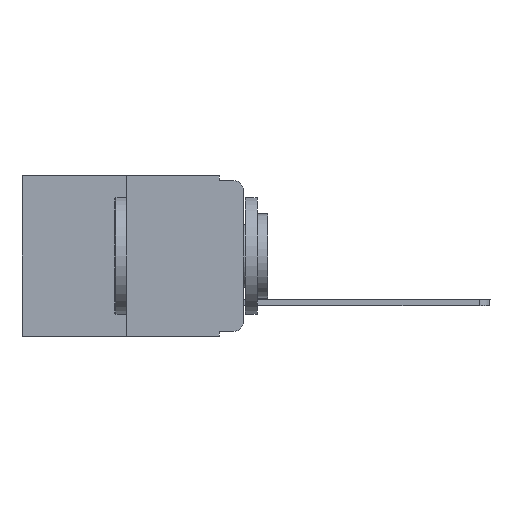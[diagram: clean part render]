
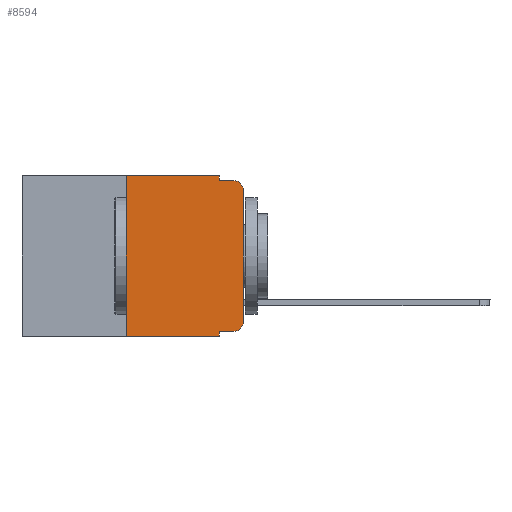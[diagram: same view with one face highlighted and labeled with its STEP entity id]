
A CAD part, left-side view. The second image highlights one B-rep face of the part: STEP entity #8594.
In plain terms, the highlighted planar face has unit normal (-1, 0, 0).
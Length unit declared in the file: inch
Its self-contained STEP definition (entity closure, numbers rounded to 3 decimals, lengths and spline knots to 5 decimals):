
#75 = EDGE_CURVE ( 'NONE', #5653, #9041, #9872, .T. ) ;
#121 = VECTOR ( 'NONE', #3713, 39.37008 ) ;
#231 = CARTESIAN_POINT ( 'NONE',  ( 0., 0.473, 0. ) ) ;
#342 = LINE ( 'NONE', #6228, #9351 ) ;
#469 = LINE ( 'NONE', #10474, #3541 ) ;
#540 = EDGE_LOOP ( 'NONE', ( #1932, #5531, #7216, #6764, #4128, #2574, #12078, #12370, #7357, #11386 ) ) ;
#544 = VERTEX_POINT ( 'NONE', #5443 ) ;
#1088 = CIRCLE ( 'NONE', #3472, 0.02 ) ;
#1161 = EDGE_CURVE ( 'NONE', #544, #10805, #2858, .T. ) ;
#1884 = EDGE_CURVE ( 'NONE', #5751, #6646, #12744, .T. ) ;
#1932 = ORIENTED_EDGE ( 'NONE', *, *, #5219, .T. ) ;
#2144 = DIRECTION ( 'NONE',  ( 0., -1., 0. ) ) ;
#2246 = FACE_OUTER_BOUND ( 'NONE', #540, .T. ) ;
#2435 = DIRECTION ( 'NONE',  ( 0., 0., -1. ) ) ;
#2471 = CARTESIAN_POINT ( 'NONE',  ( 0., 0.051, 0. ) ) ;
#2574 = ORIENTED_EDGE ( 'NONE', *, *, #8300, .F. ) ;
#2858 = LINE ( 'NONE', #5704, #10298 ) ;
#3012 = EDGE_CURVE ( 'NONE', #6087, #10805, #469, .T. ) ;
#3167 = DIRECTION ( 'NONE',  ( 0., 0., -1. ) ) ;
#3271 = EDGE_CURVE ( 'NONE', #5115, #5653, #8709, .T. ) ;
#3472 = AXIS2_PLACEMENT_3D ( 'NONE', #6667, #9539, #3167 ) ;
#3541 = VECTOR ( 'NONE', #12462, 39.37008 ) ;
#3556 = AXIS2_PLACEMENT_3D ( 'NONE', #231, #12052, #5066 ) ;
#3705 = DIRECTION ( 'NONE',  ( 0., 0., -1. ) ) ;
#3713 = DIRECTION ( 'NONE',  ( 0., 0., 1. ) ) ;
#4107 = VERTEX_POINT ( 'NONE', #9435 ) ;
#4128 = ORIENTED_EDGE ( 'NONE', *, *, #3271, .F. ) ;
#4273 = EDGE_CURVE ( 'NONE', #10976, #4107, #1088, .T. ) ;
#4589 = LINE ( 'NONE', #12578, #121 ) ;
#4745 = CARTESIAN_POINT ( 'NONE',  ( 0., 0., -0.03 ) ) ;
#5066 = DIRECTION ( 'NONE',  ( 0., 0., -1. ) ) ;
#5115 = VERTEX_POINT ( 'NONE', #12418 ) ;
#5219 = EDGE_CURVE ( 'NONE', #4107, #5751, #8588, .T. ) ;
#5395 = VECTOR ( 'NONE', #2144, 39.37008 ) ;
#5443 = CARTESIAN_POINT ( 'NONE',  ( 0., 0.051, -0.333 ) ) ;
#5473 = CARTESIAN_POINT ( 'NONE',  ( 0., 0.051, 0. ) ) ;
#5531 = ORIENTED_EDGE ( 'NONE', *, *, #1884, .T. ) ;
#5630 = DIRECTION ( 'NONE',  ( 0., -1., 0. ) ) ;
#5653 = VERTEX_POINT ( 'NONE', #2471 ) ;
#5704 = CARTESIAN_POINT ( 'NONE',  ( 0., 0.051, 0. ) ) ;
#5751 = VERTEX_POINT ( 'NONE', #4745 ) ;
#5788 = CARTESIAN_POINT ( 'NONE',  ( 0., 0., 0. ) ) ;
#6061 = DIRECTION ( 'NONE',  ( -1., 0., 0. ) ) ;
#6087 = VERTEX_POINT ( 'NONE', #11226 ) ;
#6228 = CARTESIAN_POINT ( 'NONE',  ( 0., 0.051, -0.333 ) ) ;
#6646 = VERTEX_POINT ( 'NONE', #7322 ) ;
#6667 = CARTESIAN_POINT ( 'NONE',  ( 0., 0.02, -0.313 ) ) ;
#6764 = ORIENTED_EDGE ( 'NONE', *, *, #75, .F. ) ;
#7216 = ORIENTED_EDGE ( 'NONE', *, *, #8308, .F. ) ;
#7322 = CARTESIAN_POINT ( 'NONE',  ( 0., 0.02, -0.01 ) ) ;
#7357 = ORIENTED_EDGE ( 'NONE', *, *, #11416, .T. ) ;
#7768 = DIRECTION ( 'NONE',  ( 0., 0., 1. ) ) ;
#7828 = CARTESIAN_POINT ( 'NONE',  ( 0., 0.051, -0.01 ) ) ;
#8138 = CARTESIAN_POINT ( 'NONE',  ( 0., 0.02, -0.03 ) ) ;
#8300 = EDGE_CURVE ( 'NONE', #6087, #5115, #4589, .T. ) ;
#8308 = EDGE_CURVE ( 'NONE', #9041, #6646, #9869, .T. ) ;
#8588 = LINE ( 'NONE', #5788, #11525 ) ;
#8594 = ADVANCED_FACE ( 'NONE', ( #2246 ), #9216, .F. ) ;
#8709 = LINE ( 'NONE', #8954, #5395 ) ;
#8834 = CARTESIAN_POINT ( 'NONE',  ( 0., 0.051, -0.01 ) ) ;
#8954 = CARTESIAN_POINT ( 'NONE',  ( 0., 0.473, 0. ) ) ;
#9041 = VERTEX_POINT ( 'NONE', #7828 ) ;
#9216 = PLANE ( 'NONE',  #3556 ) ;
#9247 = DIRECTION ( 'NONE',  ( 0., -1., 0. ) ) ;
#9351 = VECTOR ( 'NONE', #9247, 39.37008 ) ;
#9409 = VECTOR ( 'NONE', #2435, 39.37008 ) ;
#9435 = CARTESIAN_POINT ( 'NONE',  ( 0., 0., -0.313 ) ) ;
#9539 = DIRECTION ( 'NONE',  ( -1., 0., 0. ) ) ;
#9546 = CARTESIAN_POINT ( 'NONE',  ( 0., 0.02, -0.333 ) ) ;
#9869 = LINE ( 'NONE', #8834, #11892 ) ;
#9872 = LINE ( 'NONE', #5473, #9409 ) ;
#9943 = AXIS2_PLACEMENT_3D ( 'NONE', #8138, #6061, #11129 ) ;
#10298 = VECTOR ( 'NONE', #3705, 39.37008 ) ;
#10474 = CARTESIAN_POINT ( 'NONE',  ( 0., 0.473, -0.343 ) ) ;
#10805 = VERTEX_POINT ( 'NONE', #11581 ) ;
#10976 = VERTEX_POINT ( 'NONE', #9546 ) ;
#11129 = DIRECTION ( 'NONE',  ( 0., 0., -1. ) ) ;
#11226 = CARTESIAN_POINT ( 'NONE',  ( 0., 0.25, -0.343 ) ) ;
#11386 = ORIENTED_EDGE ( 'NONE', *, *, #4273, .T. ) ;
#11416 = EDGE_CURVE ( 'NONE', #544, #10976, #342, .T. ) ;
#11525 = VECTOR ( 'NONE', #7768, 39.37008 ) ;
#11581 = CARTESIAN_POINT ( 'NONE',  ( 0., 0.051, -0.343 ) ) ;
#11892 = VECTOR ( 'NONE', #5630, 39.37008 ) ;
#12052 = DIRECTION ( 'NONE',  ( 1., 0., 0. ) ) ;
#12078 = ORIENTED_EDGE ( 'NONE', *, *, #3012, .T. ) ;
#12370 = ORIENTED_EDGE ( 'NONE', *, *, #1161, .F. ) ;
#12418 = CARTESIAN_POINT ( 'NONE',  ( 0., 0.25, 0. ) ) ;
#12462 = DIRECTION ( 'NONE',  ( 0., -1., 0. ) ) ;
#12578 = CARTESIAN_POINT ( 'NONE',  ( 0., 0.25, 0. ) ) ;
#12744 = CIRCLE ( 'NONE', #9943, 0.02 ) ;
